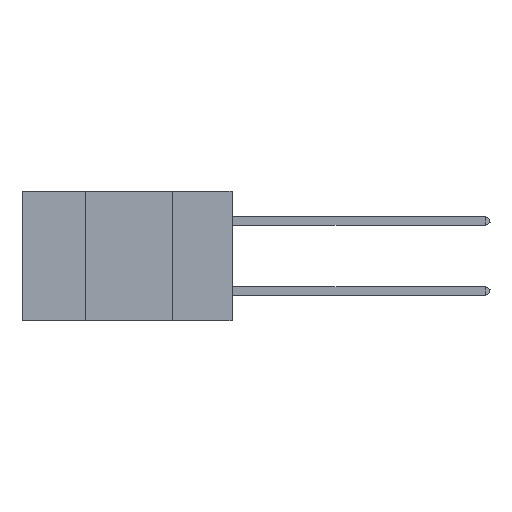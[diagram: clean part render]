
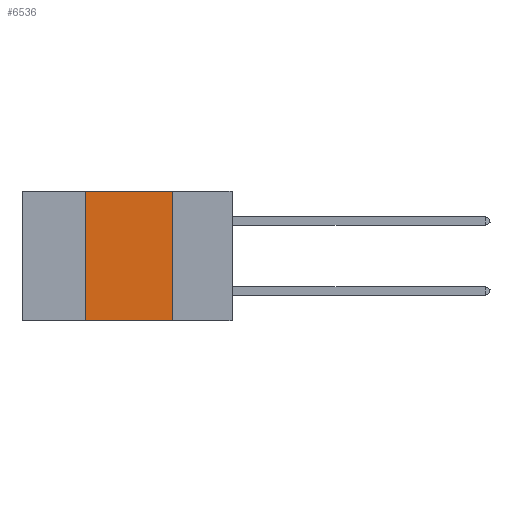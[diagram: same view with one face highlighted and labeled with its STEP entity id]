
A CAD part, left-side view. The second image highlights one B-rep face of the part: STEP entity #6536.
In plain terms, the highlighted planar face has unit normal (-1, 0, 0).
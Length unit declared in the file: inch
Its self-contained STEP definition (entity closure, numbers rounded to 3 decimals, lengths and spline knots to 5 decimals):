
#284 = DIRECTION ( 'NONE',  ( 0., -1., 0. ) ) ;
#342 = VECTOR ( 'NONE', #3601, 39.37008 ) ;
#616 = CARTESIAN_POINT ( 'NONE',  ( 0., 0.6, 0. ) ) ;
#2697 = EDGE_CURVE ( 'NONE', #22368, #22814, #23959, .T. ) ;
#3313 = ORIENTED_EDGE ( 'NONE', *, *, #2697, .F. ) ;
#3382 = ORIENTED_EDGE ( 'NONE', *, *, #14709, .T. ) ;
#3601 = DIRECTION ( 'NONE',  ( 0., 0., -1. ) ) ;
#5547 = EDGE_CURVE ( 'NONE', #13068, #22368, #12576, .T. ) ;
#6529 = CARTESIAN_POINT ( 'NONE',  ( 0., 0.6, 0. ) ) ;
#6536 = ADVANCED_FACE ( 'NONE', ( #14570 ), #27558, .F. ) ;
#6782 = DIRECTION ( 'NONE',  ( 0., -1., 0. ) ) ;
#6891 = CARTESIAN_POINT ( 'NONE',  ( 0., 0.6, -0.37 ) ) ;
#9207 = CARTESIAN_POINT ( 'NONE',  ( 0., 0.17, -0.37 ) ) ;
#9285 = CARTESIAN_POINT ( 'NONE',  ( 0., 0.17, 0. ) ) ;
#10872 = EDGE_CURVE ( 'NONE', #22814, #28591, #11949, .T. ) ;
#11454 = LINE ( 'NONE', #6891, #12274 ) ;
#11949 = LINE ( 'NONE', #9285, #342 ) ;
#12274 = VECTOR ( 'NONE', #6782, 39.37008 ) ;
#12576 = LINE ( 'NONE', #13376, #27054 ) ;
#13068 = VERTEX_POINT ( 'NONE', #23272 ) ;
#13376 = CARTESIAN_POINT ( 'NONE',  ( 0., 0.42, 0. ) ) ;
#14570 = FACE_OUTER_BOUND ( 'NONE', #33446, .T. ) ;
#14709 = EDGE_CURVE ( 'NONE', #13068, #28591, #11454, .T. ) ;
#18940 = CARTESIAN_POINT ( 'NONE',  ( 0., 0.42, 0. ) ) ;
#20824 = ORIENTED_EDGE ( 'NONE', *, *, #5547, .F. ) ;
#22368 = VERTEX_POINT ( 'NONE', #18940 ) ;
#22610 = DIRECTION ( 'NONE',  ( 0., 0., -1. ) ) ;
#22814 = VERTEX_POINT ( 'NONE', #26320 ) ;
#23272 = CARTESIAN_POINT ( 'NONE',  ( 0., 0.42, -0.37 ) ) ;
#23959 = LINE ( 'NONE', #616, #25604 ) ;
#25604 = VECTOR ( 'NONE', #284, 39.37008 ) ;
#25932 = AXIS2_PLACEMENT_3D ( 'NONE', #6529, #33538, #22610 ) ;
#26320 = CARTESIAN_POINT ( 'NONE',  ( 0., 0.17, 0. ) ) ;
#27054 = VECTOR ( 'NONE', #31956, 39.37008 ) ;
#27558 = PLANE ( 'NONE',  #25932 ) ;
#28591 = VERTEX_POINT ( 'NONE', #9207 ) ;
#30748 = ORIENTED_EDGE ( 'NONE', *, *, #10872, .F. ) ;
#31956 = DIRECTION ( 'NONE',  ( 0., 0., 1. ) ) ;
#33446 = EDGE_LOOP ( 'NONE', ( #30748, #3313, #20824, #3382 ) ) ;
#33538 = DIRECTION ( 'NONE',  ( 1., 0., 0. ) ) ;
